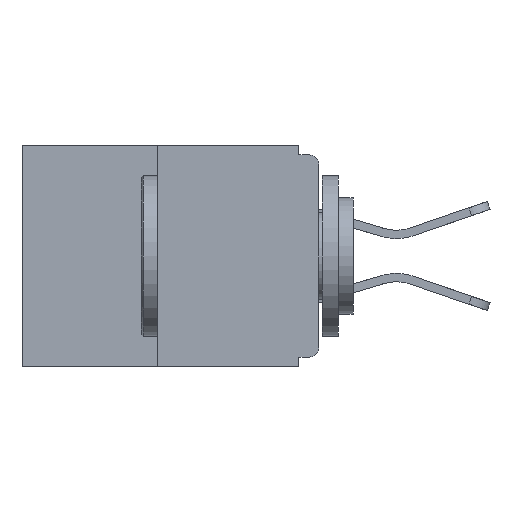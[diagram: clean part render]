
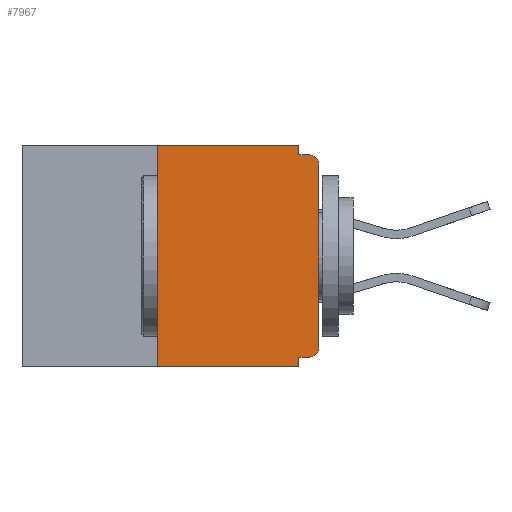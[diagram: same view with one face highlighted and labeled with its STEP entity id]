
A CAD part, left-side view. The second image highlights one B-rep face of the part: STEP entity #7967.
In plain terms, the highlighted planar face has unit normal (-1, 0, 0).
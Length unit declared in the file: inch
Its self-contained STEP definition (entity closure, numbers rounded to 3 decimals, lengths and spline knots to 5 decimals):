
#360 = AXIS2_PLACEMENT_3D ( 'NONE', #681, #17976, #12609 ) ;
#681 = CARTESIAN_POINT ( 'NONE',  ( 0., 0.015, -0.313 ) ) ;
#712 = VECTOR ( 'NONE', #8302, 39.37008 ) ;
#1147 = ORIENTED_EDGE ( 'NONE', *, *, #4962, .T. ) ;
#1528 = AXIS2_PLACEMENT_3D ( 'NONE', #16067, #9241, #21316 ) ;
#1581 = CARTESIAN_POINT ( 'NONE',  ( 0., 0.031, 0. ) ) ;
#1593 = DIRECTION ( 'NONE',  ( 0., 0., -1. ) ) ;
#1832 = ORIENTED_EDGE ( 'NONE', *, *, #9859, .T. ) ;
#2142 = EDGE_CURVE ( 'NONE', #11041, #21221, #21001, .T. ) ;
#2383 = CARTESIAN_POINT ( 'NONE',  ( 0., 0.031, -0.343 ) ) ;
#2705 = VERTEX_POINT ( 'NONE', #13616 ) ;
#2773 = VECTOR ( 'NONE', #22139, 39.37008 ) ;
#2851 = CARTESIAN_POINT ( 'NONE',  ( 0., 0., -0.015 ) ) ;
#3015 = ORIENTED_EDGE ( 'NONE', *, *, #4266, .F. ) ;
#3469 = VECTOR ( 'NONE', #5618, 39.37008 ) ;
#4207 = CARTESIAN_POINT ( 'NONE',  ( 0., 0.46, 0. ) ) ;
#4266 = EDGE_CURVE ( 'NONE', #21221, #19807, #12204, .T. ) ;
#4454 = CARTESIAN_POINT ( 'NONE',  ( 0., 0.015, -0.328 ) ) ;
#4468 = CARTESIAN_POINT ( 'NONE',  ( 0., 0., 0. ) ) ;
#4962 = EDGE_CURVE ( 'NONE', #18724, #20710, #11906, .T. ) ;
#5496 = VERTEX_POINT ( 'NONE', #7456 ) ;
#5544 = EDGE_CURVE ( 'NONE', #2705, #18452, #7597, .T. ) ;
#5614 = CARTESIAN_POINT ( 'NONE',  ( 0., 0.46, 0. ) ) ;
#5618 = DIRECTION ( 'NONE',  ( 0., 1., 0. ) ) ;
#6471 = CARTESIAN_POINT ( 'NONE',  ( 0., 0.25, -0.343 ) ) ;
#6802 = EDGE_CURVE ( 'NONE', #16282, #11041, #14577, .T. ) ;
#7149 = ORIENTED_EDGE ( 'NONE', *, *, #19925, .F. ) ;
#7314 = VECTOR ( 'NONE', #14360, 39.37008 ) ;
#7456 = CARTESIAN_POINT ( 'NONE',  ( 0., 0.015, -0.015 ) ) ;
#7468 = DIRECTION ( 'NONE',  ( 1., 0., 0. ) ) ;
#7597 = LINE ( 'NONE', #2383, #7314 ) ;
#7615 = AXIS2_PLACEMENT_3D ( 'NONE', #5614, #7468, #19353 ) ;
#7956 = CIRCLE ( 'NONE', #1528, 0.015 ) ;
#7967 = ADVANCED_FACE ( 'NONE', ( #8588 ), #11080, .F. ) ;
#8102 = EDGE_LOOP ( 'NONE', ( #13871, #12781, #9554, #15829, #7149, #9805, #1147, #1832, #8272, #3015 ) ) ;
#8272 = ORIENTED_EDGE ( 'NONE', *, *, #11056, .F. ) ;
#8302 = DIRECTION ( 'NONE',  ( 0., 0., 1. ) ) ;
#8326 = VECTOR ( 'NONE', #9195, 39.37008 ) ;
#8588 = FACE_OUTER_BOUND ( 'NONE', #8102, .T. ) ;
#8750 = EDGE_CURVE ( 'NONE', #21779, #18724, #13133, .T. ) ;
#9195 = DIRECTION ( 'NONE',  ( 0., -1., 0. ) ) ;
#9241 = DIRECTION ( 'NONE',  ( -1., 0., 0. ) ) ;
#9554 = ORIENTED_EDGE ( 'NONE', *, *, #10308, .T. ) ;
#9805 = ORIENTED_EDGE ( 'NONE', *, *, #8750, .T. ) ;
#9823 = LINE ( 'NONE', #20325, #10345 ) ;
#9859 = EDGE_CURVE ( 'NONE', #20710, #5496, #7956, .T. ) ;
#10308 = EDGE_CURVE ( 'NONE', #16282, #18452, #9823, .T. ) ;
#10312 = CARTESIAN_POINT ( 'NONE',  ( 0., 0.25, 0. ) ) ;
#10345 = VECTOR ( 'NONE', #18420, 39.37008 ) ;
#11041 = VERTEX_POINT ( 'NONE', #19763 ) ;
#11056 = EDGE_CURVE ( 'NONE', #19807, #5496, #15926, .T. ) ;
#11080 = PLANE ( 'NONE',  #7615 ) ;
#11413 = VECTOR ( 'NONE', #14832, 39.37008 ) ;
#11742 = LINE ( 'NONE', #14075, #3469 ) ;
#11906 = LINE ( 'NONE', #4468, #712 ) ;
#12204 = LINE ( 'NONE', #17073, #13305 ) ;
#12258 = CARTESIAN_POINT ( 'NONE',  ( 0., 0.031, -0.343 ) ) ;
#12609 = DIRECTION ( 'NONE',  ( 0., 0., -1. ) ) ;
#12781 = ORIENTED_EDGE ( 'NONE', *, *, #6802, .F. ) ;
#13133 = CIRCLE ( 'NONE', #360, 0.015 ) ;
#13305 = VECTOR ( 'NONE', #1593, 39.37008 ) ;
#13616 = CARTESIAN_POINT ( 'NONE',  ( 0., 0.031, -0.328 ) ) ;
#13768 = CARTESIAN_POINT ( 'NONE',  ( 0., 0.031, -0.015 ) ) ;
#13871 = ORIENTED_EDGE ( 'NONE', *, *, #2142, .F. ) ;
#14075 = CARTESIAN_POINT ( 'NONE',  ( 0., 0., -0.328 ) ) ;
#14360 = DIRECTION ( 'NONE',  ( 0., 0., -1. ) ) ;
#14459 = CARTESIAN_POINT ( 'NONE',  ( 0., 0., -0.313 ) ) ;
#14577 = LINE ( 'NONE', #10312, #2773 ) ;
#14832 = DIRECTION ( 'NONE',  ( 0., -1., 0. ) ) ;
#15829 = ORIENTED_EDGE ( 'NONE', *, *, #5544, .F. ) ;
#15926 = LINE ( 'NONE', #2851, #11413 ) ;
#16067 = CARTESIAN_POINT ( 'NONE',  ( 0., 0.015, -0.03 ) ) ;
#16282 = VERTEX_POINT ( 'NONE', #6471 ) ;
#17073 = CARTESIAN_POINT ( 'NONE',  ( 0., 0.031, 0. ) ) ;
#17976 = DIRECTION ( 'NONE',  ( -1., 0., 0. ) ) ;
#18420 = DIRECTION ( 'NONE',  ( 0., -1., 0. ) ) ;
#18452 = VERTEX_POINT ( 'NONE', #12258 ) ;
#18724 = VERTEX_POINT ( 'NONE', #14459 ) ;
#19302 = CARTESIAN_POINT ( 'NONE',  ( 0., 0., -0.03 ) ) ;
#19353 = DIRECTION ( 'NONE',  ( 0., 0., -1. ) ) ;
#19763 = CARTESIAN_POINT ( 'NONE',  ( 0., 0.25, 0. ) ) ;
#19807 = VERTEX_POINT ( 'NONE', #13768 ) ;
#19925 = EDGE_CURVE ( 'NONE', #21779, #2705, #11742, .T. ) ;
#20325 = CARTESIAN_POINT ( 'NONE',  ( 0., 0.46, -0.343 ) ) ;
#20710 = VERTEX_POINT ( 'NONE', #19302 ) ;
#21001 = LINE ( 'NONE', #4207, #8326 ) ;
#21221 = VERTEX_POINT ( 'NONE', #1581 ) ;
#21316 = DIRECTION ( 'NONE',  ( 0., 0., -1. ) ) ;
#21779 = VERTEX_POINT ( 'NONE', #4454 ) ;
#22139 = DIRECTION ( 'NONE',  ( 0., 0., 1. ) ) ;
